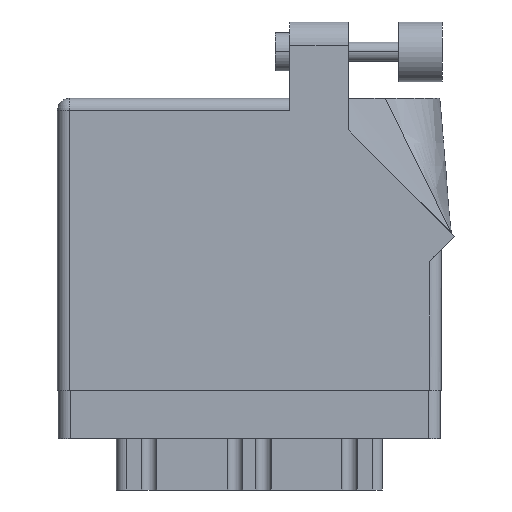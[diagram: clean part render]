
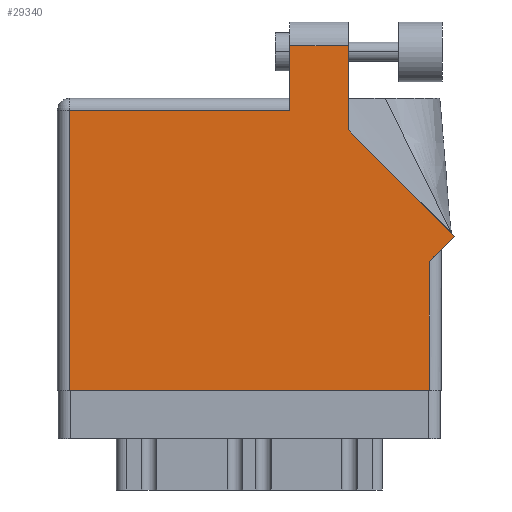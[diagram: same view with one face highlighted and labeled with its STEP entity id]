
A CAD part, front view. The second image highlights one B-rep face of the part: STEP entity #29340.
In plain terms, the highlighted face is planar.
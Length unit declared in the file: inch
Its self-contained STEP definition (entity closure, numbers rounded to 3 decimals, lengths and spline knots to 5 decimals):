
#280 = ORIENTED_EDGE ( 'NONE', *, *, #4408, .T. ) ;
#2375 = LINE ( 'NONE', #20259, #24341 ) ;
#2700 = DIRECTION ( 'NONE',  ( 0., 0., -1. ) ) ;
#2746 = CARTESIAN_POINT ( 'NONE',  ( 1.948, 0.737, 0. ) ) ;
#3409 = CARTESIAN_POINT ( 'NONE',  ( 1.217, 1.805, 0. ) ) ;
#3917 = ORIENTED_EDGE ( 'NONE', *, *, #32121, .T. ) ;
#4408 = EDGE_CURVE ( 'NONE', #32267, #7084, #2375, .T. ) ;
#7080 = DIRECTION ( 'NONE',  ( 0., -1., 0. ) ) ;
#7084 = VERTEX_POINT ( 'NONE', #24515 ) ;
#8515 = CARTESIAN_POINT ( 'NONE',  ( 0., 1.53, 0. ) ) ;
#9403 = CARTESIAN_POINT ( 'NONE',  ( 1.217, 1.53, 0. ) ) ;
#10135 = ORIENTED_EDGE ( 'NONE', *, *, #24890, .T. ) ;
#10566 = CARTESIAN_POINT ( 'NONE',  ( 2.01, 0.737, 0. ) ) ;
#10633 = VERTEX_POINT ( 'NONE', #31589 ) ;
#10893 = EDGE_CURVE ( 'NONE', #11305, #23621, #30849, .T. ) ;
#11305 = VERTEX_POINT ( 'NONE', #27976 ) ;
#12223 = LINE ( 'NONE', #9403, #34955 ) ;
#13399 = LINE ( 'NONE', #10566, #30463 ) ;
#13510 = DIRECTION ( 'NONE',  ( 0., 1., 0. ) ) ;
#13527 = VECTOR ( 'NONE', #29246, 39.37008 ) ;
#13557 = VECTOR ( 'NONE', #17269, 39.37008 ) ;
#15606 = ORIENTED_EDGE ( 'NONE', *, *, #28958, .T. ) ;
#16738 = ORIENTED_EDGE ( 'NONE', *, *, #10893, .T. ) ;
#16899 = CARTESIAN_POINT ( 'NONE',  ( 0.062, 0., 0. ) ) ;
#16965 = DIRECTION ( 'NONE',  ( -1., 0., 0. ) ) ;
#17092 = CARTESIAN_POINT ( 'NONE',  ( 1.217, 1.805, 0. ) ) ;
#17269 = DIRECTION ( 'NONE',  ( 0., 1., 0. ) ) ;
#18005 = VERTEX_POINT ( 'NONE', #30077 ) ;
#18275 = ORIENTED_EDGE ( 'NONE', *, *, #25602, .T. ) ;
#18466 = CARTESIAN_POINT ( 'NONE',  ( 2.08071, 0.80771, 0. ) ) ;
#18599 = ORIENTED_EDGE ( 'NONE', *, *, #26295, .T. ) ;
#19288 = DIRECTION ( 'NONE',  ( -1., 0., 0. ) ) ;
#19600 = LINE ( 'NONE', #30371, #20237 ) ;
#20095 = CARTESIAN_POINT ( 'NONE',  ( 1.217, 1.468, 0. ) ) ;
#20237 = VECTOR ( 'NONE', #16965, 39.37008 ) ;
#20259 = CARTESIAN_POINT ( 'NONE',  ( 0., 0., 0. ) ) ;
#20511 = LINE ( 'NONE', #31273, #34850 ) ;
#20602 = AXIS2_PLACEMENT_3D ( 'NONE', #8515, #2700, #19288 ) ;
#21011 = VERTEX_POINT ( 'NONE', #20095 ) ;
#21120 = LINE ( 'NONE', #18466, #13527 ) ;
#21345 = DIRECTION ( 'NONE',  ( 0.707, 0.707, 0. ) ) ;
#22866 = CARTESIAN_POINT ( 'NONE',  ( 1.524, 1.36442, 0. ) ) ;
#23621 = VERTEX_POINT ( 'NONE', #3409 ) ;
#24051 = DIRECTION ( 'NONE',  ( 1., 0., 0. ) ) ;
#24341 = VECTOR ( 'NONE', #24051, 39.37008 ) ;
#24483 = EDGE_CURVE ( 'NONE', #23621, #21011, #12223, .T. ) ;
#24504 = VECTOR ( 'NONE', #13510, 39.37008 ) ;
#24515 = CARTESIAN_POINT ( 'NONE',  ( 1.948, 0., 0. ) ) ;
#24890 = EDGE_CURVE ( 'NONE', #21011, #10633, #19600, .T. ) ;
#25602 = EDGE_CURVE ( 'NONE', #18005, #26953, #21120, .T. ) ;
#26295 = EDGE_CURVE ( 'NONE', #28862, #18005, #13399, .T. ) ;
#26375 = EDGE_CURVE ( 'NONE', #26953, #11305, #32823, .T. ) ;
#26953 = VERTEX_POINT ( 'NONE', #22866 ) ;
#27976 = CARTESIAN_POINT ( 'NONE',  ( 1.524, 1.805, 0. ) ) ;
#28350 = EDGE_LOOP ( 'NONE', ( #32089, #16738, #33431, #10135, #3917, #280, #15606, #18599, #18275 ) ) ;
#28390 = DIRECTION ( 'NONE',  ( -1., 0., 0. ) ) ;
#28862 = VERTEX_POINT ( 'NONE', #32505 ) ;
#28958 = EDGE_CURVE ( 'NONE', #7084, #28862, #32559, .T. ) ;
#29246 = DIRECTION ( 'NONE',  ( -0.707, 0.707, 0. ) ) ;
#29340 = ADVANCED_FACE ( 'NONE', ( #29364 ), #32707, .F. ) ;
#29364 = FACE_OUTER_BOUND ( 'NONE', #28350, .T. ) ;
#30077 = CARTESIAN_POINT ( 'NONE',  ( 2.08071, 0.80771, 0. ) ) ;
#30371 = CARTESIAN_POINT ( 'NONE',  ( 0., 1.468, 0. ) ) ;
#30463 = VECTOR ( 'NONE', #21345, 39.37008 ) ;
#30694 = CARTESIAN_POINT ( 'NONE',  ( 1.524, 1.36442, 0. ) ) ;
#30849 = LINE ( 'NONE', #17092, #30995 ) ;
#30948 = DIRECTION ( 'NONE',  ( 0., -1., 0. ) ) ;
#30995 = VECTOR ( 'NONE', #28390, 39.37008 ) ;
#31273 = CARTESIAN_POINT ( 'NONE',  ( 0.062, 0., 0. ) ) ;
#31589 = CARTESIAN_POINT ( 'NONE',  ( 0.062, 1.468, 0. ) ) ;
#32089 = ORIENTED_EDGE ( 'NONE', *, *, #26375, .T. ) ;
#32121 = EDGE_CURVE ( 'NONE', #10633, #32267, #20511, .T. ) ;
#32267 = VERTEX_POINT ( 'NONE', #16899 ) ;
#32505 = CARTESIAN_POINT ( 'NONE',  ( 1.948, 0.675, 0. ) ) ;
#32559 = LINE ( 'NONE', #2746, #24504 ) ;
#32707 = PLANE ( 'NONE',  #20602 ) ;
#32823 = LINE ( 'NONE', #30694, #13557 ) ;
#33431 = ORIENTED_EDGE ( 'NONE', *, *, #24483, .T. ) ;
#34850 = VECTOR ( 'NONE', #7080, 39.37008 ) ;
#34955 = VECTOR ( 'NONE', #30948, 39.37008 ) ;
